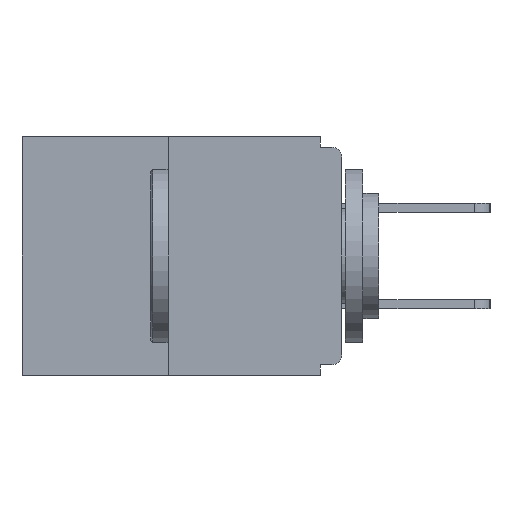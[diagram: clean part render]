
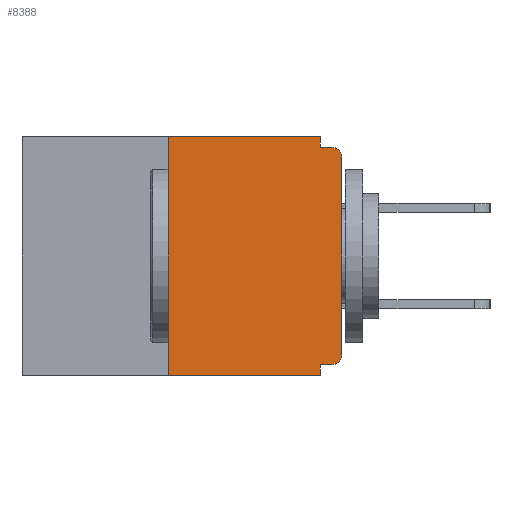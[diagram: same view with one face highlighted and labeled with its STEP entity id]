
A CAD part, left-side view. The second image highlights one B-rep face of the part: STEP entity #8388.
In plain terms, the highlighted planar face has unit normal (-1, 0, 0).
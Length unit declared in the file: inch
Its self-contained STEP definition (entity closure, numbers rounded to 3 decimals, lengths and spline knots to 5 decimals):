
#108 = FACE_OUTER_BOUND ( 'NONE', #19396, .T. ) ;
#268 = EDGE_CURVE ( 'NONE', #18629, #6062, #19954, .T. ) ;
#505 = DIRECTION ( 'NONE',  ( 0., 0., -1. ) ) ;
#1117 = ORIENTED_EDGE ( 'NONE', *, *, #268, .F. ) ;
#1898 = EDGE_CURVE ( 'NONE', #20627, #16006, #6114, .T. ) ;
#2013 = DIRECTION ( 'NONE',  ( 0., -1., 0. ) ) ;
#2188 = DIRECTION ( 'NONE',  ( 0., 1., 0. ) ) ;
#2845 = AXIS2_PLACEMENT_3D ( 'NONE', #4567, #17864, #505 ) ;
#2879 = CARTESIAN_POINT ( 'NONE',  ( 0., 0., -0.015 ) ) ;
#3347 = EDGE_CURVE ( 'NONE', #9480, #20627, #16094, .T. ) ;
#3465 = VECTOR ( 'NONE', #2013, 39.37008 ) ;
#3530 = CARTESIAN_POINT ( 'NONE',  ( 0., 0.25, -0.343 ) ) ;
#3936 = LINE ( 'NONE', #15201, #18855 ) ;
#4567 = CARTESIAN_POINT ( 'NONE',  ( 0., 0.46, 0. ) ) ;
#4697 = DIRECTION ( 'NONE',  ( 0., 0., -1. ) ) ;
#5435 = DIRECTION ( 'NONE',  ( 0., -1., 0. ) ) ;
#5582 = EDGE_CURVE ( 'NONE', #10456, #22086, #16893, .T. ) ;
#5763 = EDGE_CURVE ( 'NONE', #10456, #10699, #8651, .T. ) ;
#5923 = VECTOR ( 'NONE', #12621, 39.37008 ) ;
#6062 = VERTEX_POINT ( 'NONE', #11183 ) ;
#6114 = LINE ( 'NONE', #23503, #15866 ) ;
#6520 = LINE ( 'NONE', #11928, #22998 ) ;
#7088 = CARTESIAN_POINT ( 'NONE',  ( 0., 0.031, -0.328 ) ) ;
#7182 = ORIENTED_EDGE ( 'NONE', *, *, #11171, .F. ) ;
#8088 = EDGE_CURVE ( 'NONE', #11994, #22086, #20578, .T. ) ;
#8388 = ADVANCED_FACE ( 'NONE', ( #108 ), #21948, .F. ) ;
#8538 = ORIENTED_EDGE ( 'NONE', *, *, #5582, .T. ) ;
#8651 = LINE ( 'NONE', #13251, #10188 ) ;
#8801 = ORIENTED_EDGE ( 'NONE', *, *, #10404, .F. ) ;
#9197 = AXIS2_PLACEMENT_3D ( 'NONE', #19209, #23243, #23148 ) ;
#9480 = VERTEX_POINT ( 'NONE', #13395 ) ;
#10188 = VECTOR ( 'NONE', #11455, 39.37008 ) ;
#10287 = ORIENTED_EDGE ( 'NONE', *, *, #5763, .F. ) ;
#10404 = EDGE_CURVE ( 'NONE', #11930, #18629, #10713, .T. ) ;
#10456 = VERTEX_POINT ( 'NONE', #3530 ) ;
#10593 = CARTESIAN_POINT ( 'NONE',  ( 0., 0.015, -0.03 ) ) ;
#10699 = VERTEX_POINT ( 'NONE', #20899 ) ;
#10713 = LINE ( 'NONE', #20467, #16796 ) ;
#11171 = EDGE_CURVE ( 'NONE', #10699, #11930, #3936, .T. ) ;
#11183 = CARTESIAN_POINT ( 'NONE',  ( 0., 0.015, -0.015 ) ) ;
#11248 = ORIENTED_EDGE ( 'NONE', *, *, #15532, .T. ) ;
#11443 = AXIS2_PLACEMENT_3D ( 'NONE', #10593, #14491, #24228 ) ;
#11455 = DIRECTION ( 'NONE',  ( 0., 0., 1. ) ) ;
#11758 = CARTESIAN_POINT ( 'NONE',  ( 0., 0., -0.313 ) ) ;
#11919 = CARTESIAN_POINT ( 'NONE',  ( 0., 0.46, -0.343 ) ) ;
#11928 = CARTESIAN_POINT ( 'NONE',  ( 0., 0., -0.328 ) ) ;
#11930 = VERTEX_POINT ( 'NONE', #22028 ) ;
#11994 = VERTEX_POINT ( 'NONE', #7088 ) ;
#12621 = DIRECTION ( 'NONE',  ( 0., -1., 0. ) ) ;
#12671 = EDGE_CURVE ( 'NONE', #9480, #11994, #6520, .T. ) ;
#12684 = ORIENTED_EDGE ( 'NONE', *, *, #1898, .T. ) ;
#13251 = CARTESIAN_POINT ( 'NONE',  ( 0., 0.25, 0. ) ) ;
#13395 = CARTESIAN_POINT ( 'NONE',  ( 0., 0.015, -0.328 ) ) ;
#14491 = DIRECTION ( 'NONE',  ( -1., 0., 0. ) ) ;
#15115 = DIRECTION ( 'NONE',  ( 0., 0., 1. ) ) ;
#15201 = CARTESIAN_POINT ( 'NONE',  ( 0., 0.46, 0. ) ) ;
#15532 = EDGE_CURVE ( 'NONE', #16006, #6062, #16768, .T. ) ;
#15866 = VECTOR ( 'NONE', #15115, 39.37008 ) ;
#16006 = VERTEX_POINT ( 'NONE', #16295 ) ;
#16021 = VECTOR ( 'NONE', #19752, 39.37008 ) ;
#16094 = CIRCLE ( 'NONE', #9197, 0.015 ) ;
#16295 = CARTESIAN_POINT ( 'NONE',  ( 0., 0., -0.03 ) ) ;
#16436 = ORIENTED_EDGE ( 'NONE', *, *, #3347, .T. ) ;
#16768 = CIRCLE ( 'NONE', #11443, 0.015 ) ;
#16796 = VECTOR ( 'NONE', #4697, 39.37008 ) ;
#16893 = LINE ( 'NONE', #11919, #3465 ) ;
#17864 = DIRECTION ( 'NONE',  ( 1., 0., 0. ) ) ;
#18115 = CARTESIAN_POINT ( 'NONE',  ( 0., 0.031, -0.343 ) ) ;
#18504 = CARTESIAN_POINT ( 'NONE',  ( 0., 0.031, -0.015 ) ) ;
#18629 = VERTEX_POINT ( 'NONE', #18504 ) ;
#18855 = VECTOR ( 'NONE', #5435, 39.37008 ) ;
#18859 = ORIENTED_EDGE ( 'NONE', *, *, #8088, .F. ) ;
#19209 = CARTESIAN_POINT ( 'NONE',  ( 0., 0.015, -0.313 ) ) ;
#19396 = EDGE_LOOP ( 'NONE', ( #7182, #10287, #8538, #18859, #22992, #16436, #12684, #11248, #1117, #8801 ) ) ;
#19752 = DIRECTION ( 'NONE',  ( 0., 0., -1. ) ) ;
#19954 = LINE ( 'NONE', #2879, #5923 ) ;
#20467 = CARTESIAN_POINT ( 'NONE',  ( 0., 0.031, 0. ) ) ;
#20578 = LINE ( 'NONE', #18115, #16021 ) ;
#20627 = VERTEX_POINT ( 'NONE', #11758 ) ;
#20899 = CARTESIAN_POINT ( 'NONE',  ( 0., 0.25, 0. ) ) ;
#21948 = PLANE ( 'NONE',  #2845 ) ;
#22028 = CARTESIAN_POINT ( 'NONE',  ( 0., 0.031, 0. ) ) ;
#22086 = VERTEX_POINT ( 'NONE', #22616 ) ;
#22616 = CARTESIAN_POINT ( 'NONE',  ( 0., 0.031, -0.343 ) ) ;
#22992 = ORIENTED_EDGE ( 'NONE', *, *, #12671, .F. ) ;
#22998 = VECTOR ( 'NONE', #2188, 39.37008 ) ;
#23148 = DIRECTION ( 'NONE',  ( 0., 0., -1. ) ) ;
#23243 = DIRECTION ( 'NONE',  ( -1., 0., 0. ) ) ;
#23503 = CARTESIAN_POINT ( 'NONE',  ( 0., 0., 0. ) ) ;
#24228 = DIRECTION ( 'NONE',  ( 0., 0., -1. ) ) ;
